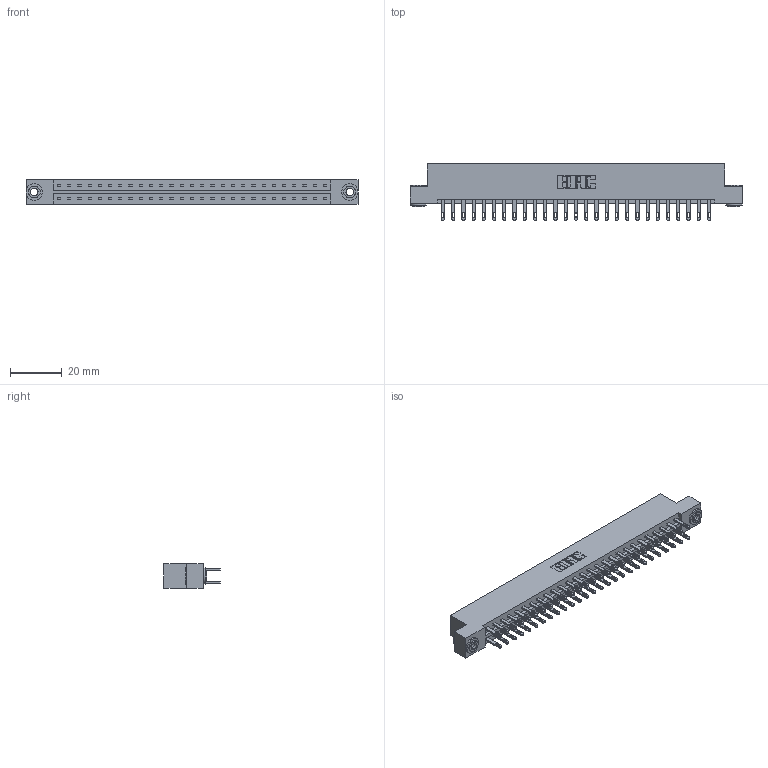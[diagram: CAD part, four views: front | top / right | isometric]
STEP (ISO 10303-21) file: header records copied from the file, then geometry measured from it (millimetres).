
FILE_DESCRIPTION (( 'STEP AP203' ), '1' );
FILE_NAME ('833-054-500-203.STEP', '2020-06-04T20:15:00', ( '' ), ( '' ), 'SwSTEP 2.0', 'SolidWorks 2020', '' );
FILE_SCHEMA (( 'CONFIG_CONTROL_DESIGN' ));
Length unit declared in the file: inch
Products named in the file (4): 345-292-001_345-293-100; 833 Part_Flush - .156 Dia - TH; 345-250-002_345-250-002-102; 833-054-500-203
Assembly tree (57 placements, depth 2):
  833-054-500-203
    833 Part_Flush - .156 Dia - TH
    345-292-001_345-293-100  x54
    345-250-002_345-250-002-102  x2
Bounding box: 128.52 x 21.85 x 9.4 mm (x, y, z)
Volume: 13165.7 mm3; surface area: 16219.1 mm2
Topology: 57 solids, 57 shells, 2744 faces, 8325 edges, 5546 vertices
Faces by surface type: plane 1700, cylinder 1036, cone 8
Entity records: 19890 total; most frequent: CARTESIAN_POINT 3289, ORIENTED_EDGE 3218, DIRECTION 2871, EDGE_CURVE 1609, LINE 1453, VECTOR 1453, VERTEX_POINT 1070, AXIS2_PLACEMENT_3D 709
